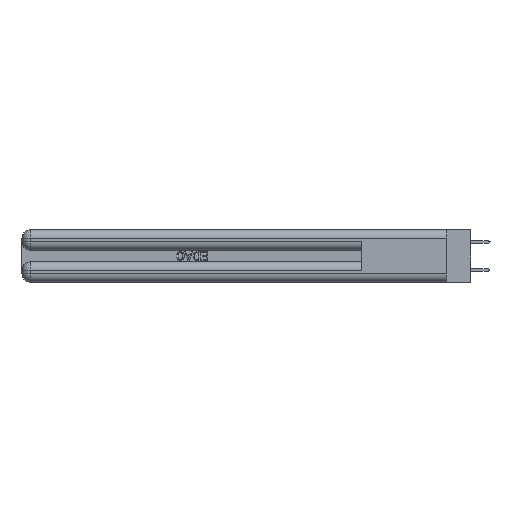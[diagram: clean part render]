
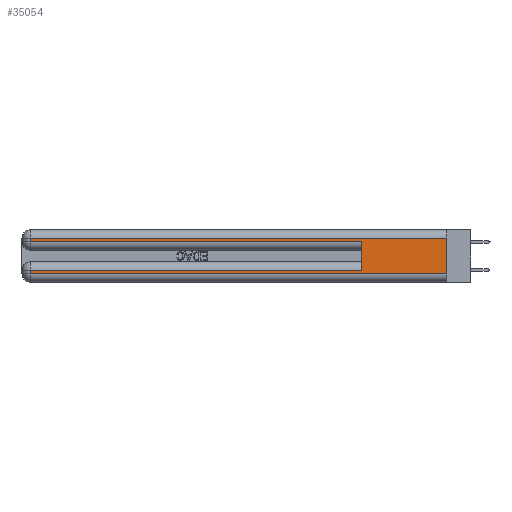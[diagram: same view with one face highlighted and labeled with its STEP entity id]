
A CAD part, left-side view. The second image highlights one B-rep face of the part: STEP entity #35054.
In plain terms, the highlighted planar face has unit normal (-1, 0, 0).
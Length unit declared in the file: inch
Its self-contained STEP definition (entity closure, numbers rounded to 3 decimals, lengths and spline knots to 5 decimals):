
#667 = LINE ( 'NONE', #21201, #50168 ) ;
#1248 = VECTOR ( 'NONE', #44361, 39.37008 ) ;
#1547 = CARTESIAN_POINT ( 'NONE',  ( 0., 0., 0.285 ) ) ;
#2342 = VECTOR ( 'NONE', #17933, 39.37008 ) ;
#5072 = CARTESIAN_POINT ( 'NONE',  ( 0., 2.94, 0.31 ) ) ;
#5529 = EDGE_CURVE ( 'NONE', #34723, #33586, #7502, .T. ) ;
#6123 = EDGE_CURVE ( 'NONE', #33586, #21639, #33402, .T. ) ;
#6993 = DIRECTION ( 'NONE',  ( 0., 1., 0. ) ) ;
#7261 = EDGE_CURVE ( 'NONE', #28780, #38853, #17616, .T. ) ;
#7502 = LINE ( 'NONE', #23055, #45813 ) ;
#8536 = CARTESIAN_POINT ( 'NONE',  ( 0., 0., 0.06 ) ) ;
#9679 = EDGE_CURVE ( 'NONE', #37439, #20032, #667, .T. ) ;
#11456 = DIRECTION ( 'NONE',  ( 0., 0., -1. ) ) ;
#11580 = EDGE_CURVE ( 'NONE', #11882, #28780, #46110, .T. ) ;
#11882 = VERTEX_POINT ( 'NONE', #45007 ) ;
#12235 = EDGE_LOOP ( 'NONE', ( #33743, #20102, #47763, #32655, #20416, #43621, #36112, #38274 ) ) ;
#13154 = DIRECTION ( 'NONE',  ( 0., 0., -1. ) ) ;
#16732 = DIRECTION ( 'NONE',  ( 0., 0., -1. ) ) ;
#17616 = LINE ( 'NONE', #49760, #42422 ) ;
#17933 = DIRECTION ( 'NONE',  ( 0., 1., 0. ) ) ;
#19621 = LINE ( 'NONE', #51760, #43707 ) ;
#20032 = VERTEX_POINT ( 'NONE', #8536 ) ;
#20102 = ORIENTED_EDGE ( 'NONE', *, *, #21210, .T. ) ;
#20416 = ORIENTED_EDGE ( 'NONE', *, *, #28597, .F. ) ;
#20809 = FACE_OUTER_BOUND ( 'NONE', #12235, .T. ) ;
#21201 = CARTESIAN_POINT ( 'NONE',  ( 0., 0., 0.37 ) ) ;
#21210 = EDGE_CURVE ( 'NONE', #37439, #34723, #19621, .T. ) ;
#21639 = VERTEX_POINT ( 'NONE', #39301 ) ;
#23055 = CARTESIAN_POINT ( 'NONE',  ( 0., 2.94, 0.37 ) ) ;
#24100 = CARTESIAN_POINT ( 'NONE',  ( 0., 0.6, 0.145 ) ) ;
#24234 = PLANE ( 'NONE',  #33349 ) ;
#27198 = VECTOR ( 'NONE', #44751, 39.37008 ) ;
#28436 = CARTESIAN_POINT ( 'NONE',  ( 0., 0., 0.37 ) ) ;
#28597 = EDGE_CURVE ( 'NONE', #11882, #21639, #31988, .T. ) ;
#28780 = VERTEX_POINT ( 'NONE', #38011 ) ;
#31988 = LINE ( 'NONE', #24100, #1248 ) ;
#32400 = DIRECTION ( 'NONE',  ( 0., 0., -1. ) ) ;
#32655 = ORIENTED_EDGE ( 'NONE', *, *, #6123, .T. ) ;
#33349 = AXIS2_PLACEMENT_3D ( 'NONE', #28436, #44505, #32400 ) ;
#33402 = LINE ( 'NONE', #1547, #27198 ) ;
#33586 = VERTEX_POINT ( 'NONE', #48195 ) ;
#33743 = ORIENTED_EDGE ( 'NONE', *, *, #9679, .F. ) ;
#34350 = CARTESIAN_POINT ( 'NONE',  ( 0., 2.94, 0.06 ) ) ;
#34723 = VERTEX_POINT ( 'NONE', #5072 ) ;
#35054 = ADVANCED_FACE ( 'NONE', ( #20809 ), #24234, .F. ) ;
#36112 = ORIENTED_EDGE ( 'NONE', *, *, #7261, .T. ) ;
#37164 = EDGE_CURVE ( 'NONE', #38853, #20032, #41797, .T. ) ;
#37439 = VERTEX_POINT ( 'NONE', #40705 ) ;
#38011 = CARTESIAN_POINT ( 'NONE',  ( 0., 2.94, 0.085 ) ) ;
#38105 = DIRECTION ( 'NONE',  ( 0., -1., 0. ) ) ;
#38274 = ORIENTED_EDGE ( 'NONE', *, *, #37164, .T. ) ;
#38459 = CARTESIAN_POINT ( 'NONE',  ( 0., 0., 0.085 ) ) ;
#38540 = VECTOR ( 'NONE', #38105, 39.37008 ) ;
#38853 = VERTEX_POINT ( 'NONE', #34350 ) ;
#39301 = CARTESIAN_POINT ( 'NONE',  ( 0., 0.6, 0.285 ) ) ;
#40705 = CARTESIAN_POINT ( 'NONE',  ( 0., 0., 0.31 ) ) ;
#41797 = LINE ( 'NONE', #46536, #38540 ) ;
#42422 = VECTOR ( 'NONE', #13154, 39.37008 ) ;
#43621 = ORIENTED_EDGE ( 'NONE', *, *, #11580, .T. ) ;
#43707 = VECTOR ( 'NONE', #6993, 39.37008 ) ;
#44361 = DIRECTION ( 'NONE',  ( 0., 0., 1. ) ) ;
#44505 = DIRECTION ( 'NONE',  ( 1., 0., 0. ) ) ;
#44751 = DIRECTION ( 'NONE',  ( 0., -1., 0. ) ) ;
#45007 = CARTESIAN_POINT ( 'NONE',  ( 0., 0.6, 0.085 ) ) ;
#45813 = VECTOR ( 'NONE', #11456, 39.37008 ) ;
#46110 = LINE ( 'NONE', #38459, #2342 ) ;
#46536 = CARTESIAN_POINT ( 'NONE',  ( 0., 0., 0.06 ) ) ;
#47763 = ORIENTED_EDGE ( 'NONE', *, *, #5529, .T. ) ;
#48195 = CARTESIAN_POINT ( 'NONE',  ( 0., 2.94, 0.285 ) ) ;
#49760 = CARTESIAN_POINT ( 'NONE',  ( 0., 2.94, 0.37 ) ) ;
#50168 = VECTOR ( 'NONE', #16732, 39.37008 ) ;
#51760 = CARTESIAN_POINT ( 'NONE',  ( 0., 0., 0.31 ) ) ;
